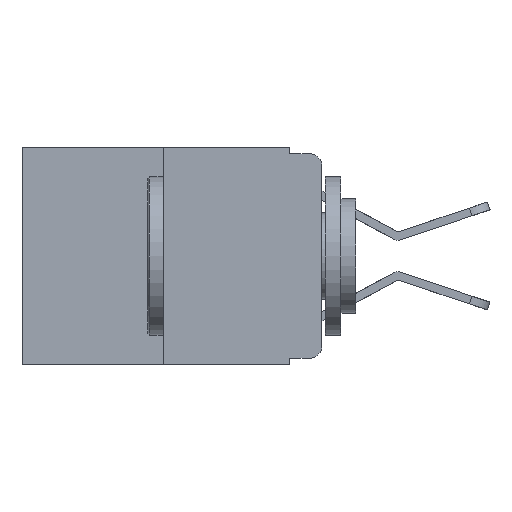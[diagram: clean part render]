
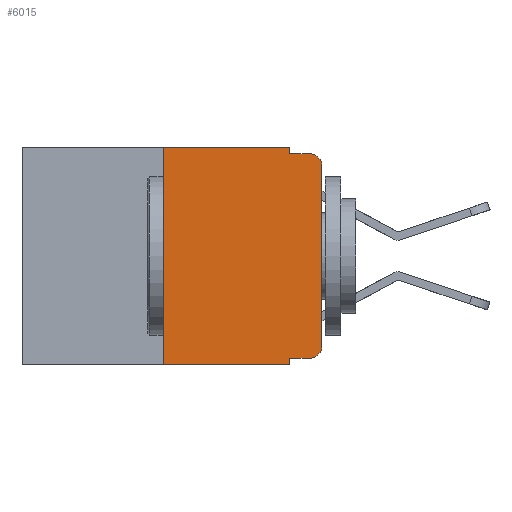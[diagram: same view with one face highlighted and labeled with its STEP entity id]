
A CAD part, left-side view. The second image highlights one B-rep face of the part: STEP entity #6015.
In plain terms, the highlighted planar face has unit normal (-1, 0, 0).
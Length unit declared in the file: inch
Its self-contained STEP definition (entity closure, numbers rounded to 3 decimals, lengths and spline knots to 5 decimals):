
#3 = CARTESIAN_POINT ( 'NONE',  ( 0., 0.051, -0.333 ) ) ;
#695 = DIRECTION ( 'NONE',  ( -1., 0., 0. ) ) ;
#938 = CARTESIAN_POINT ( 'NONE',  ( 0., 0.25, -0.343 ) ) ;
#1342 = ORIENTED_EDGE ( 'NONE', *, *, #13241, .T. ) ;
#1811 = VECTOR ( 'NONE', #20419, 39.37008 ) ;
#1843 = CARTESIAN_POINT ( 'NONE',  ( 0., 0., -0.313 ) ) ;
#2079 = ORIENTED_EDGE ( 'NONE', *, *, #9811, .F. ) ;
#2195 = CARTESIAN_POINT ( 'NONE',  ( 0., 0.473, -0.343 ) ) ;
#2214 = ORIENTED_EDGE ( 'NONE', *, *, #8665, .F. ) ;
#2570 = DIRECTION ( 'NONE',  ( -1., 0., 0. ) ) ;
#2579 = ORIENTED_EDGE ( 'NONE', *, *, #5711, .F. ) ;
#3053 = EDGE_CURVE ( 'NONE', #20760, #17184, #19292, .T. ) ;
#3798 = CARTESIAN_POINT ( 'NONE',  ( 0., 0.02, -0.01 ) ) ;
#3814 = CARTESIAN_POINT ( 'NONE',  ( 0., 0.25, 0. ) ) ;
#3875 = DIRECTION ( 'NONE',  ( 0., -1., 0. ) ) ;
#4037 = ORIENTED_EDGE ( 'NONE', *, *, #6385, .F. ) ;
#4159 = CARTESIAN_POINT ( 'NONE',  ( 0., 0., -0.03 ) ) ;
#4747 = ORIENTED_EDGE ( 'NONE', *, *, #21162, .T. ) ;
#5267 = EDGE_CURVE ( 'NONE', #20760, #6271, #15262, .T. ) ;
#5473 = VECTOR ( 'NONE', #15294, 39.37008 ) ;
#5711 = EDGE_CURVE ( 'NONE', #14877, #9978, #15741, .T. ) ;
#5745 = FACE_OUTER_BOUND ( 'NONE', #10514, .T. ) ;
#6015 = ADVANCED_FACE ( 'NONE', ( #5745 ), #16305, .F. ) ;
#6222 = DIRECTION ( 'NONE',  ( 1., 0., 0. ) ) ;
#6271 = VERTEX_POINT ( 'NONE', #20200 ) ;
#6385 = EDGE_CURVE ( 'NONE', #15417, #14877, #19551, .T. ) ;
#7036 = VECTOR ( 'NONE', #18532, 39.37008 ) ;
#7722 = LINE ( 'NONE', #16244, #19449 ) ;
#7807 = CARTESIAN_POINT ( 'NONE',  ( 0., 0.051, -0.01 ) ) ;
#8665 = EDGE_CURVE ( 'NONE', #9978, #12717, #7722, .T. ) ;
#9450 = CARTESIAN_POINT ( 'NONE',  ( 0., 0.051, -0.01 ) ) ;
#9534 = DIRECTION ( 'NONE',  ( 0., -1., 0. ) ) ;
#9811 = EDGE_CURVE ( 'NONE', #12717, #18329, #20743, .T. ) ;
#9978 = VERTEX_POINT ( 'NONE', #19905 ) ;
#10514 = EDGE_LOOP ( 'NONE', ( #13983, #1342, #2079, #2214, #2579, #4037, #4747, #10660, #13108, #15316 ) ) ;
#10660 = ORIENTED_EDGE ( 'NONE', *, *, #5267, .F. ) ;
#10792 = VECTOR ( 'NONE', #11088, 39.37008 ) ;
#10854 = CARTESIAN_POINT ( 'NONE',  ( 0., 0.02, -0.03 ) ) ;
#11088 = DIRECTION ( 'NONE',  ( 0., 0., -1. ) ) ;
#11220 = DIRECTION ( 'NONE',  ( 0., 0., -1. ) ) ;
#11673 = VECTOR ( 'NONE', #3875, 39.37008 ) ;
#11845 = VERTEX_POINT ( 'NONE', #1843 ) ;
#12006 = VECTOR ( 'NONE', #9534, 39.37008 ) ;
#12261 = DIRECTION ( 'NONE',  ( 0., -1., 0. ) ) ;
#12547 = DIRECTION ( 'NONE',  ( 0., 0., -1. ) ) ;
#12645 = CARTESIAN_POINT ( 'NONE',  ( 0., 0.02, -0.313 ) ) ;
#12649 = AXIS2_PLACEMENT_3D ( 'NONE', #10854, #695, #12547 ) ;
#12708 = CARTESIAN_POINT ( 'NONE',  ( 0., 0.02, -0.333 ) ) ;
#12717 = VERTEX_POINT ( 'NONE', #9450 ) ;
#12950 = CARTESIAN_POINT ( 'NONE',  ( 0., 0.25, 0. ) ) ;
#13108 = ORIENTED_EDGE ( 'NONE', *, *, #3053, .T. ) ;
#13241 = EDGE_CURVE ( 'NONE', #21271, #18329, #16530, .T. ) ;
#13709 = AXIS2_PLACEMENT_3D ( 'NONE', #21132, #6222, #17924 ) ;
#13983 = ORIENTED_EDGE ( 'NONE', *, *, #14338, .T. ) ;
#14338 = EDGE_CURVE ( 'NONE', #11845, #21271, #20331, .T. ) ;
#14343 = DIRECTION ( 'NONE',  ( 0., 0., -1. ) ) ;
#14877 = VERTEX_POINT ( 'NONE', #12950 ) ;
#15087 = AXIS2_PLACEMENT_3D ( 'NONE', #12645, #2570, #14343 ) ;
#15239 = VECTOR ( 'NONE', #12261, 39.37008 ) ;
#15262 = LINE ( 'NONE', #17666, #10792 ) ;
#15294 = DIRECTION ( 'NONE',  ( 0., -1., 0. ) ) ;
#15316 = ORIENTED_EDGE ( 'NONE', *, *, #21286, .T. ) ;
#15417 = VERTEX_POINT ( 'NONE', #938 ) ;
#15598 = CARTESIAN_POINT ( 'NONE',  ( 0., 0.473, 0. ) ) ;
#15741 = LINE ( 'NONE', #15598, #15239 ) ;
#16076 = CARTESIAN_POINT ( 'NONE',  ( 0., 0.051, -0.333 ) ) ;
#16244 = CARTESIAN_POINT ( 'NONE',  ( 0., 0.051, 0. ) ) ;
#16305 = PLANE ( 'NONE',  #13709 ) ;
#16530 = CIRCLE ( 'NONE', #12649, 0.02 ) ;
#16925 = CARTESIAN_POINT ( 'NONE',  ( 0., 0., 0. ) ) ;
#17184 = VERTEX_POINT ( 'NONE', #12708 ) ;
#17666 = CARTESIAN_POINT ( 'NONE',  ( 0., 0.051, 0. ) ) ;
#17844 = CIRCLE ( 'NONE', #15087, 0.02 ) ;
#17924 = DIRECTION ( 'NONE',  ( 0., 0., -1. ) ) ;
#18329 = VERTEX_POINT ( 'NONE', #3798 ) ;
#18532 = DIRECTION ( 'NONE',  ( 0., 0., 1. ) ) ;
#19292 = LINE ( 'NONE', #3, #5473 ) ;
#19449 = VECTOR ( 'NONE', #11220, 39.37008 ) ;
#19551 = LINE ( 'NONE', #3814, #1811 ) ;
#19905 = CARTESIAN_POINT ( 'NONE',  ( 0., 0.051, 0. ) ) ;
#20200 = CARTESIAN_POINT ( 'NONE',  ( 0., 0.051, -0.343 ) ) ;
#20331 = LINE ( 'NONE', #16925, #7036 ) ;
#20417 = LINE ( 'NONE', #2195, #11673 ) ;
#20419 = DIRECTION ( 'NONE',  ( 0., 0., 1. ) ) ;
#20743 = LINE ( 'NONE', #7807, #12006 ) ;
#20760 = VERTEX_POINT ( 'NONE', #16076 ) ;
#21132 = CARTESIAN_POINT ( 'NONE',  ( 0., 0.473, 0. ) ) ;
#21162 = EDGE_CURVE ( 'NONE', #15417, #6271, #20417, .T. ) ;
#21271 = VERTEX_POINT ( 'NONE', #4159 ) ;
#21286 = EDGE_CURVE ( 'NONE', #17184, #11845, #17844, .T. ) ;
